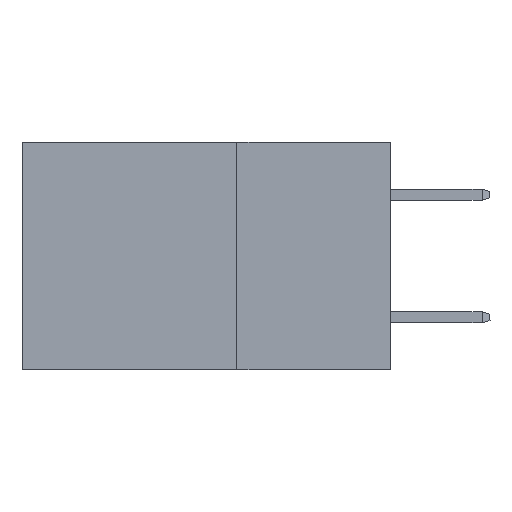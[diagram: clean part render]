
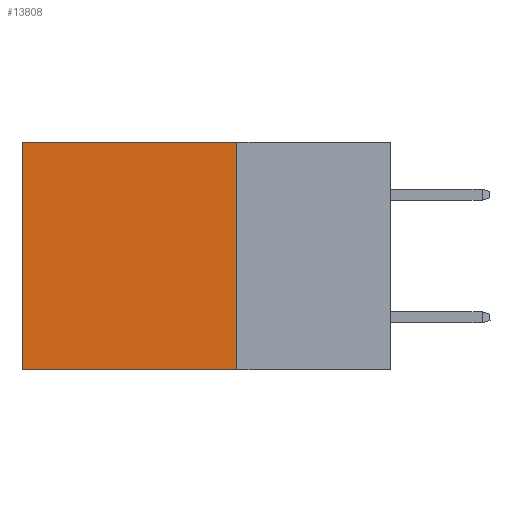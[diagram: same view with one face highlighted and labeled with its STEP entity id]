
A CAD part, left-side view. The second image highlights one B-rep face of the part: STEP entity #13808.
In plain terms, the highlighted planar face has unit normal (-1, 0, 0).
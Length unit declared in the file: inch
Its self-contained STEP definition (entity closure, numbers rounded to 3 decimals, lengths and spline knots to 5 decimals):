
#2019 = VECTOR ( 'NONE', #4131, 39.37008 ) ;
#2577 = CARTESIAN_POINT ( 'NONE',  ( 0.2875, 0.6, 0. ) ) ;
#2950 = CARTESIAN_POINT ( 'NONE',  ( 0.2875, 0.25, 0. ) ) ;
#3085 = DIRECTION ( 'NONE',  ( 0., 0., -1. ) ) ;
#3097 = CARTESIAN_POINT ( 'NONE',  ( 0.2875, 0.25, -0.37 ) ) ;
#3370 = VERTEX_POINT ( 'NONE', #3097 ) ;
#3654 = ORIENTED_EDGE ( 'NONE', *, *, #12816, .F. ) ;
#4131 = DIRECTION ( 'NONE',  ( 0., 0., -1. ) ) ;
#4954 = DIRECTION ( 'NONE',  ( 0., 1., 0. ) ) ;
#7613 = EDGE_CURVE ( 'NONE', #15857, #3370, #8529, .T. ) ;
#8204 = VERTEX_POINT ( 'NONE', #16958 ) ;
#8312 = PLANE ( 'NONE',  #18429 ) ;
#8529 = LINE ( 'NONE', #10553, #11552 ) ;
#8901 = DIRECTION ( 'NONE',  ( 0., 1., 0. ) ) ;
#9080 = FACE_OUTER_BOUND ( 'NONE', #18508, .T. ) ;
#9737 = CARTESIAN_POINT ( 'NONE',  ( 0.2875, 0.25, 0. ) ) ;
#9741 = CARTESIAN_POINT ( 'NONE',  ( 0.2875, 0.25, 0. ) ) ;
#9797 = DIRECTION ( 'NONE',  ( 0., 0., -1. ) ) ;
#10553 = CARTESIAN_POINT ( 'NONE',  ( 0.2875, 0.25, 0. ) ) ;
#10985 = VECTOR ( 'NONE', #4954, 39.37008 ) ;
#11498 = VERTEX_POINT ( 'NONE', #12416 ) ;
#11552 = VECTOR ( 'NONE', #3085, 39.37008 ) ;
#11924 = ORIENTED_EDGE ( 'NONE', *, *, #18261, .T. ) ;
#12123 = VECTOR ( 'NONE', #8901, 39.37008 ) ;
#12416 = CARTESIAN_POINT ( 'NONE',  ( 0.2875, 0.6, -0.37 ) ) ;
#12816 = EDGE_CURVE ( 'NONE', #3370, #11498, #14989, .T. ) ;
#13808 = ADVANCED_FACE ( 'NONE', ( #9080 ), #8312, .F. ) ;
#13937 = LINE ( 'NONE', #2577, #2019 ) ;
#14667 = EDGE_CURVE ( 'NONE', #8204, #11498, #13937, .T. ) ;
#14989 = LINE ( 'NONE', #15468, #10985 ) ;
#15194 = LINE ( 'NONE', #2950, #12123 ) ;
#15468 = CARTESIAN_POINT ( 'NONE',  ( 0.2875, 0.25, -0.37 ) ) ;
#15857 = VERTEX_POINT ( 'NONE', #9737 ) ;
#16559 = ORIENTED_EDGE ( 'NONE', *, *, #14667, .T. ) ;
#16958 = CARTESIAN_POINT ( 'NONE',  ( 0.2875, 0.6, 0. ) ) ;
#17848 = ORIENTED_EDGE ( 'NONE', *, *, #7613, .F. ) ;
#18261 = EDGE_CURVE ( 'NONE', #15857, #8204, #15194, .T. ) ;
#18429 = AXIS2_PLACEMENT_3D ( 'NONE', #9741, #18805, #9797 ) ;
#18508 = EDGE_LOOP ( 'NONE', ( #16559, #3654, #17848, #11924 ) ) ;
#18805 = DIRECTION ( 'NONE',  ( 1., 0., 0. ) ) ;
